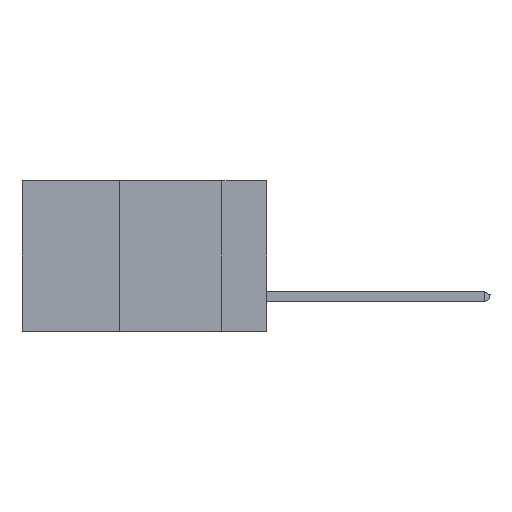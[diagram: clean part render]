
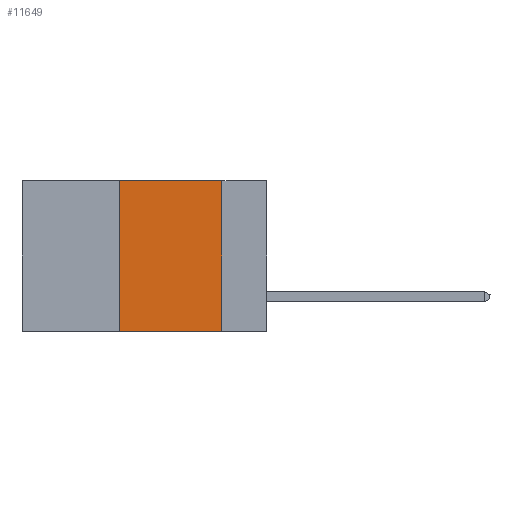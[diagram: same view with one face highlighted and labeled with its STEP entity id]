
A CAD part, left-side view. The second image highlights one B-rep face of the part: STEP entity #11649.
In plain terms, the highlighted planar face has unit normal (-1, 0, 0).
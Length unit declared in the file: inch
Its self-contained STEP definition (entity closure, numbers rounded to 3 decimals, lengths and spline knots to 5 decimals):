
#953 = VECTOR ( 'NONE', #12343, 39.37008 ) ;
#1279 = LINE ( 'NONE', #4048, #24890 ) ;
#1574 = DIRECTION ( 'NONE',  ( 0., 0., -1. ) ) ;
#1965 = DIRECTION ( 'NONE',  ( 0., 0., -1. ) ) ;
#2027 = DIRECTION ( 'NONE',  ( 0., 0., 1. ) ) ;
#3698 = EDGE_CURVE ( 'NONE', #13462, #20508, #25202, .T. ) ;
#4014 = ORIENTED_EDGE ( 'NONE', *, *, #12695, .F. ) ;
#4048 = CARTESIAN_POINT ( 'NONE',  ( 0., 0.6, -0.37 ) ) ;
#4066 = CARTESIAN_POINT ( 'NONE',  ( 0., 0.36, 0. ) ) ;
#4665 = VERTEX_POINT ( 'NONE', #16511 ) ;
#4710 = CARTESIAN_POINT ( 'NONE',  ( 0., 0.11, 0. ) ) ;
#5867 = PLANE ( 'NONE',  #21093 ) ;
#6331 = CARTESIAN_POINT ( 'NONE',  ( 0., 0.36, 0. ) ) ;
#9791 = EDGE_CURVE ( 'NONE', #13462, #4665, #1279, .T. ) ;
#10692 = EDGE_LOOP ( 'NONE', ( #19097, #4014, #28051, #18428 ) ) ;
#11649 = ADVANCED_FACE ( 'NONE', ( #18275 ), #5867, .F. ) ;
#12343 = DIRECTION ( 'NONE',  ( 0., -1., 0. ) ) ;
#12695 = EDGE_CURVE ( 'NONE', #20508, #25525, #29050, .T. ) ;
#13462 = VERTEX_POINT ( 'NONE', #21988 ) ;
#13739 = VECTOR ( 'NONE', #1965, 39.37008 ) ;
#13756 = VECTOR ( 'NONE', #2027, 39.37008 ) ;
#15223 = CARTESIAN_POINT ( 'NONE',  ( 0., 0.6, 0. ) ) ;
#15408 = DIRECTION ( 'NONE',  ( 0., -1., 0. ) ) ;
#15921 = LINE ( 'NONE', #4710, #13739 ) ;
#16511 = CARTESIAN_POINT ( 'NONE',  ( 0., 0.11, -0.37 ) ) ;
#18275 = FACE_OUTER_BOUND ( 'NONE', #10692, .T. ) ;
#18428 = ORIENTED_EDGE ( 'NONE', *, *, #9791, .T. ) ;
#19097 = ORIENTED_EDGE ( 'NONE', *, *, #21314, .F. ) ;
#20508 = VERTEX_POINT ( 'NONE', #4066 ) ;
#21093 = AXIS2_PLACEMENT_3D ( 'NONE', #15223, #22580, #1574 ) ;
#21314 = EDGE_CURVE ( 'NONE', #25525, #4665, #15921, .T. ) ;
#21988 = CARTESIAN_POINT ( 'NONE',  ( 0., 0.36, -0.37 ) ) ;
#22580 = DIRECTION ( 'NONE',  ( 1., 0., 0. ) ) ;
#24784 = CARTESIAN_POINT ( 'NONE',  ( 0., 0.11, 0. ) ) ;
#24890 = VECTOR ( 'NONE', #15408, 39.37008 ) ;
#25202 = LINE ( 'NONE', #6331, #13756 ) ;
#25525 = VERTEX_POINT ( 'NONE', #24784 ) ;
#26730 = CARTESIAN_POINT ( 'NONE',  ( 0., 0.6, 0. ) ) ;
#28051 = ORIENTED_EDGE ( 'NONE', *, *, #3698, .F. ) ;
#29050 = LINE ( 'NONE', #26730, #953 ) ;
